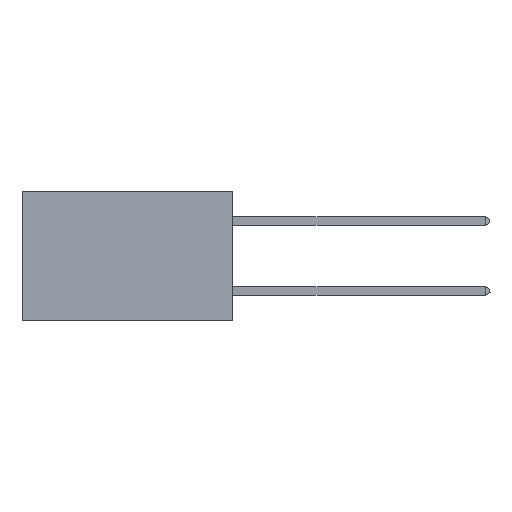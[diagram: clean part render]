
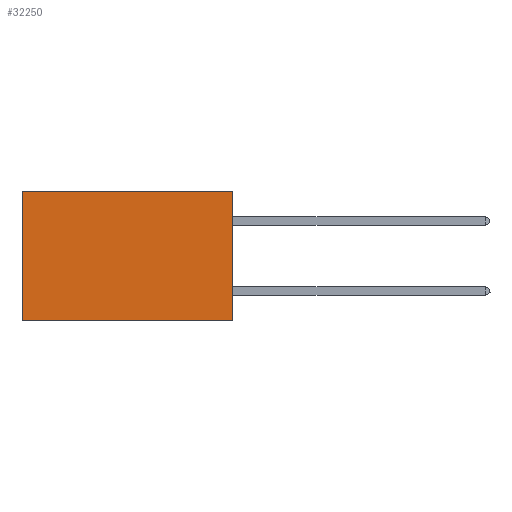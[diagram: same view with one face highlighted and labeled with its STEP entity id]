
A CAD part, left-side view. The second image highlights one B-rep face of the part: STEP entity #32250.
In plain terms, the highlighted planar face has unit normal (-1, 0, 0).
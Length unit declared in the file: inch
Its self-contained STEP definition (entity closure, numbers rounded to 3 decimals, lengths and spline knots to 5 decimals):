
#38 = ORIENTED_EDGE ( 'NONE', *, *, #15947, .T. ) ;
#387 = VERTEX_POINT ( 'NONE', #7891 ) ;
#807 = CARTESIAN_POINT ( 'NONE',  ( 0.2875, 0., 0. ) ) ;
#1073 = CARTESIAN_POINT ( 'NONE',  ( 0.2875, 0., 0. ) ) ;
#1191 = AXIS2_PLACEMENT_3D ( 'NONE', #21864, #33280, #4769 ) ;
#3527 = VECTOR ( 'NONE', #21085, 39.37008 ) ;
#4769 = DIRECTION ( 'NONE',  ( 0., 0., -1. ) ) ;
#7211 = VECTOR ( 'NONE', #8153, 39.37008 ) ;
#7891 = CARTESIAN_POINT ( 'NONE',  ( 0.2875, 0., 0. ) ) ;
#8153 = DIRECTION ( 'NONE',  ( 0., 0., -1. ) ) ;
#10455 = PLANE ( 'NONE',  #1191 ) ;
#11087 = VECTOR ( 'NONE', #36808, 39.37008 ) ;
#11143 = CARTESIAN_POINT ( 'NONE',  ( 0.2875, 0., -0.37 ) ) ;
#12292 = LINE ( 'NONE', #807, #24479 ) ;
#12910 = CARTESIAN_POINT ( 'NONE',  ( 0.2875, 0.6, 0. ) ) ;
#13440 = ORIENTED_EDGE ( 'NONE', *, *, #30707, .F. ) ;
#13489 = LINE ( 'NONE', #31201, #7211 ) ;
#13592 = VERTEX_POINT ( 'NONE', #11143 ) ;
#15577 = ORIENTED_EDGE ( 'NONE', *, *, #30122, .T. ) ;
#15947 = EDGE_CURVE ( 'NONE', #387, #23005, #12292, .T. ) ;
#16142 = LINE ( 'NONE', #1073, #3527 ) ;
#17225 = CARTESIAN_POINT ( 'NONE',  ( 0.2875, 0.6, -0.37 ) ) ;
#19150 = VERTEX_POINT ( 'NONE', #17225 ) ;
#21085 = DIRECTION ( 'NONE',  ( 0., 0., -1. ) ) ;
#21864 = CARTESIAN_POINT ( 'NONE',  ( 0.2875, 0., 0. ) ) ;
#23005 = VERTEX_POINT ( 'NONE', #12910 ) ;
#24479 = VECTOR ( 'NONE', #29606, 39.37008 ) ;
#27170 = EDGE_CURVE ( 'NONE', #13592, #19150, #37172, .T. ) ;
#27558 = EDGE_LOOP ( 'NONE', ( #15577, #33491, #13440, #38 ) ) ;
#28495 = CARTESIAN_POINT ( 'NONE',  ( 0.2875, 0., -0.37 ) ) ;
#29545 = FACE_OUTER_BOUND ( 'NONE', #27558, .T. ) ;
#29606 = DIRECTION ( 'NONE',  ( 0., 1., 0. ) ) ;
#30122 = EDGE_CURVE ( 'NONE', #23005, #19150, #13489, .T. ) ;
#30707 = EDGE_CURVE ( 'NONE', #387, #13592, #16142, .T. ) ;
#31201 = CARTESIAN_POINT ( 'NONE',  ( 0.2875, 0.6, 0. ) ) ;
#32250 = ADVANCED_FACE ( 'NONE', ( #29545 ), #10455, .F. ) ;
#33280 = DIRECTION ( 'NONE',  ( 1., 0., 0. ) ) ;
#33491 = ORIENTED_EDGE ( 'NONE', *, *, #27170, .F. ) ;
#36808 = DIRECTION ( 'NONE',  ( 0., 1., 0. ) ) ;
#37172 = LINE ( 'NONE', #28495, #11087 ) ;
